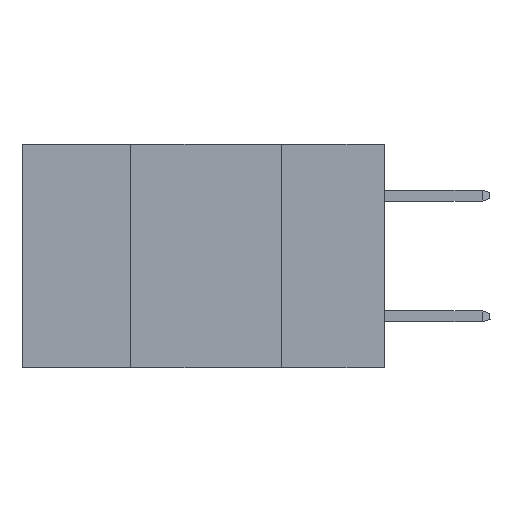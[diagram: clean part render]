
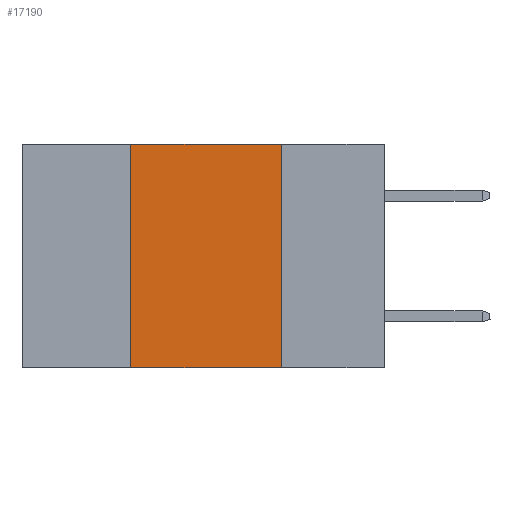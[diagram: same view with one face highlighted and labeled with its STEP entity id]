
A CAD part, left-side view. The second image highlights one B-rep face of the part: STEP entity #17190.
In plain terms, the highlighted planar face has unit normal (-1, 0, 0).
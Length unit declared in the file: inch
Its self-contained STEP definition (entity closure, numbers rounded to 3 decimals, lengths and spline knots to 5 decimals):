
#853 = EDGE_CURVE ( 'NONE', #6531, #14005, #14733, .T. ) ;
#940 = ORIENTED_EDGE ( 'NONE', *, *, #2306, .F. ) ;
#973 = EDGE_CURVE ( 'NONE', #7127, #14005, #4683, .T. ) ;
#1268 = DIRECTION ( 'NONE',  ( 0., 0., 1. ) ) ;
#1436 = CARTESIAN_POINT ( 'NONE',  ( 0., 0.42, -0.37 ) ) ;
#1561 = DIRECTION ( 'NONE',  ( 1., 0., 0. ) ) ;
#1974 = CARTESIAN_POINT ( 'NONE',  ( 0., 0.17, 0. ) ) ;
#2306 = EDGE_CURVE ( 'NONE', #13971, #6531, #13459, .T. ) ;
#2348 = CARTESIAN_POINT ( 'NONE',  ( 0., 0.42, -0.37 ) ) ;
#2584 = VECTOR ( 'NONE', #10100, 39.37008 ) ;
#2632 = AXIS2_PLACEMENT_3D ( 'NONE', #10702, #1561, #12231 ) ;
#4683 = LINE ( 'NONE', #7604, #8264 ) ;
#6326 = EDGE_CURVE ( 'NONE', #7127, #13971, #11190, .T. ) ;
#6531 = VERTEX_POINT ( 'NONE', #1974 ) ;
#7127 = VERTEX_POINT ( 'NONE', #2348 ) ;
#7604 = CARTESIAN_POINT ( 'NONE',  ( 0., 0.6, -0.37 ) ) ;
#8036 = DIRECTION ( 'NONE',  ( 0., -1., 0. ) ) ;
#8264 = VECTOR ( 'NONE', #8036, 39.37008 ) ;
#10100 = DIRECTION ( 'NONE',  ( 0., 0., -1. ) ) ;
#10171 = CARTESIAN_POINT ( 'NONE',  ( 0., 0.17, -0.37 ) ) ;
#10654 = PLANE ( 'NONE',  #2632 ) ;
#10702 = CARTESIAN_POINT ( 'NONE',  ( 0., 0.6, 0. ) ) ;
#11190 = LINE ( 'NONE', #1436, #18268 ) ;
#12231 = DIRECTION ( 'NONE',  ( 0., 0., -1. ) ) ;
#13440 = ORIENTED_EDGE ( 'NONE', *, *, #973, .T. ) ;
#13459 = LINE ( 'NONE', #19228, #16538 ) ;
#13643 = EDGE_LOOP ( 'NONE', ( #13904, #940, #18563, #13440 ) ) ;
#13904 = ORIENTED_EDGE ( 'NONE', *, *, #853, .F. ) ;
#13971 = VERTEX_POINT ( 'NONE', #14885 ) ;
#14005 = VERTEX_POINT ( 'NONE', #17951 ) ;
#14733 = LINE ( 'NONE', #10171, #2584 ) ;
#14885 = CARTESIAN_POINT ( 'NONE',  ( 0., 0.42, 0. ) ) ;
#16538 = VECTOR ( 'NONE', #19262, 39.37008 ) ;
#17190 = ADVANCED_FACE ( 'NONE', ( #18294 ), #10654, .F. ) ;
#17951 = CARTESIAN_POINT ( 'NONE',  ( 0., 0.17, -0.37 ) ) ;
#18268 = VECTOR ( 'NONE', #1268, 39.37008 ) ;
#18294 = FACE_OUTER_BOUND ( 'NONE', #13643, .T. ) ;
#18563 = ORIENTED_EDGE ( 'NONE', *, *, #6326, .F. ) ;
#19228 = CARTESIAN_POINT ( 'NONE',  ( 0., 0.6, 0. ) ) ;
#19262 = DIRECTION ( 'NONE',  ( 0., -1., 0. ) ) ;
